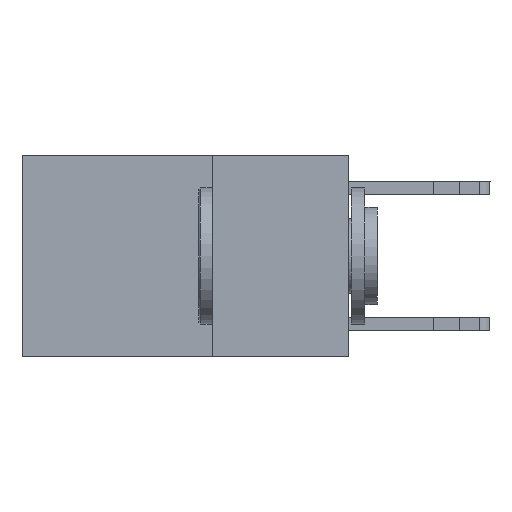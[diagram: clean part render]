
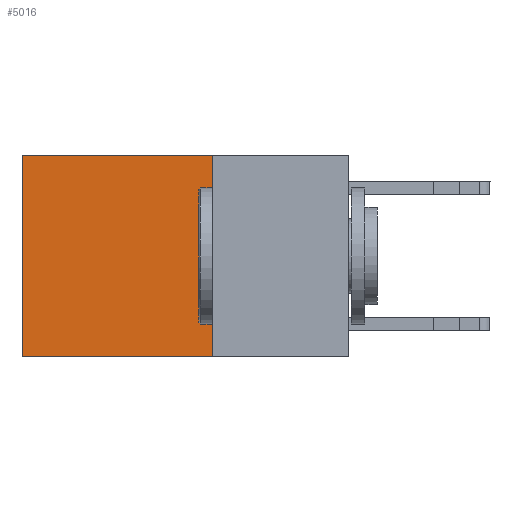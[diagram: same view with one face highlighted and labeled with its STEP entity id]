
A CAD part, left-side view. The second image highlights one B-rep face of the part: STEP entity #5016.
In plain terms, the highlighted planar face has unit normal (-1, 0, 0).
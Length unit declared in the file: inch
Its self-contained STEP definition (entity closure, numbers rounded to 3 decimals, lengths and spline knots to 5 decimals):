
#237 = CARTESIAN_POINT ( 'NONE',  ( 0.2625, 0.6, 0. ) ) ;
#924 = EDGE_LOOP ( 'NONE', ( #1994, #22657, #12463, #21020 ) ) ;
#1660 = CARTESIAN_POINT ( 'NONE',  ( 0.2625, 0.25, 0. ) ) ;
#1994 = ORIENTED_EDGE ( 'NONE', *, *, #6118, .T. ) ;
#3304 = CARTESIAN_POINT ( 'NONE',  ( 0.2625, 0.6, -0.37 ) ) ;
#3340 = CARTESIAN_POINT ( 'NONE',  ( 0.2625, 0.6, 0. ) ) ;
#3798 = EDGE_CURVE ( 'NONE', #6780, #6610, #7373, .T. ) ;
#4649 = CARTESIAN_POINT ( 'NONE',  ( 0.2625, 0.25, 0. ) ) ;
#4770 = DIRECTION ( 'NONE',  ( 0., 0., -1. ) ) ;
#5016 = ADVANCED_FACE ( 'NONE', ( #23197 ), #10671, .F. ) ;
#5192 = VERTEX_POINT ( 'NONE', #3304 ) ;
#6118 = EDGE_CURVE ( 'NONE', #6610, #5192, #21638, .T. ) ;
#6610 = VERTEX_POINT ( 'NONE', #237 ) ;
#6780 = VERTEX_POINT ( 'NONE', #23301 ) ;
#7373 = LINE ( 'NONE', #1660, #18144 ) ;
#9479 = EDGE_CURVE ( 'NONE', #9826, #5192, #19153, .T. ) ;
#9677 = DIRECTION ( 'NONE',  ( 0., 1., 0. ) ) ;
#9826 = VERTEX_POINT ( 'NONE', #12560 ) ;
#10671 = PLANE ( 'NONE',  #17805 ) ;
#10709 = CARTESIAN_POINT ( 'NONE',  ( 0.2625, 0.25, -0.37 ) ) ;
#10972 = DIRECTION ( 'NONE',  ( 0., 1., 0. ) ) ;
#11486 = DIRECTION ( 'NONE',  ( 0., 0., -1. ) ) ;
#12463 = ORIENTED_EDGE ( 'NONE', *, *, #24835, .F. ) ;
#12560 = CARTESIAN_POINT ( 'NONE',  ( 0.2625, 0.25, -0.37 ) ) ;
#12904 = DIRECTION ( 'NONE',  ( 0., 0., -1. ) ) ;
#17805 = AXIS2_PLACEMENT_3D ( 'NONE', #4649, #21059, #4770 ) ;
#18144 = VECTOR ( 'NONE', #9677, 39.37008 ) ;
#18528 = VECTOR ( 'NONE', #12904, 39.37008 ) ;
#19153 = LINE ( 'NONE', #10709, #20093 ) ;
#20093 = VECTOR ( 'NONE', #10972, 39.37008 ) ;
#20615 = VECTOR ( 'NONE', #11486, 39.37008 ) ;
#21020 = ORIENTED_EDGE ( 'NONE', *, *, #3798, .T. ) ;
#21059 = DIRECTION ( 'NONE',  ( 1., 0., 0. ) ) ;
#21638 = LINE ( 'NONE', #3340, #20615 ) ;
#22657 = ORIENTED_EDGE ( 'NONE', *, *, #9479, .F. ) ;
#23051 = CARTESIAN_POINT ( 'NONE',  ( 0.2625, 0.25, 0. ) ) ;
#23197 = FACE_OUTER_BOUND ( 'NONE', #924, .T. ) ;
#23301 = CARTESIAN_POINT ( 'NONE',  ( 0.2625, 0.25, 0. ) ) ;
#24835 = EDGE_CURVE ( 'NONE', #6780, #9826, #25056, .T. ) ;
#25056 = LINE ( 'NONE', #23051, #18528 ) ;
